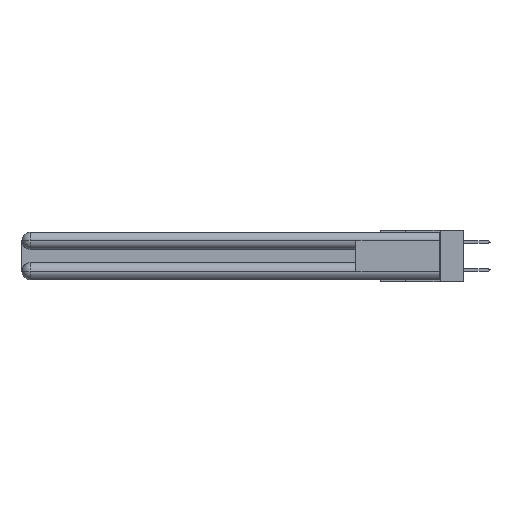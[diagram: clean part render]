
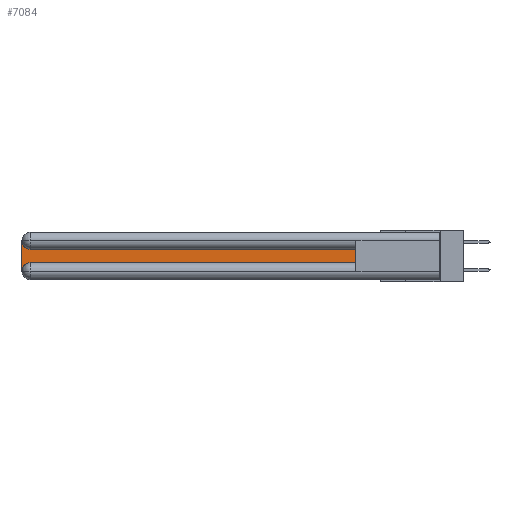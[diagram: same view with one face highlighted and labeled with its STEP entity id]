
A CAD part, left-side view. The second image highlights one B-rep face of the part: STEP entity #7084.
In plain terms, the highlighted planar face has unit normal (-1, 0, 0).
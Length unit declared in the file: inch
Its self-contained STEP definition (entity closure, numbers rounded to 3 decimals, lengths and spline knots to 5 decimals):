
#772 = ORIENTED_EDGE ( 'NONE', *, *, #11521, .T. ) ;
#3946 = VECTOR ( 'NONE', #28432, 39.37008 ) ;
#5142 = CIRCLE ( 'NONE', #7296, 0.06 ) ;
#6500 = DIRECTION ( 'NONE',  ( 0., 1., 0. ) ) ;
#7084 = ADVANCED_FACE ( 'NONE', ( #16347 ), #7309, .F. ) ;
#7296 = AXIS2_PLACEMENT_3D ( 'NONE', #9101, #19307, #32123 ) ;
#7309 = PLANE ( 'NONE',  #29893 ) ;
#7628 = EDGE_LOOP ( 'NONE', ( #17224, #16325, #29909, #25573, #772, #27453 ) ) ;
#9101 = CARTESIAN_POINT ( 'NONE',  ( 0.075, 2.94, -0.0625 ) ) ;
#9223 = EDGE_CURVE ( 'NONE', #13386, #19911, #5142, .T. ) ;
#9277 = EDGE_CURVE ( 'NONE', #19240, #13386, #19748, .T. ) ;
#9415 = EDGE_CURVE ( 'NONE', #11434, #25570, #26625, .T. ) ;
#9767 = CARTESIAN_POINT ( 'NONE',  ( 0.075, 0.6, -0.2175 ) ) ;
#10267 = VECTOR ( 'NONE', #27916, 39.37008 ) ;
#11434 = VERTEX_POINT ( 'NONE', #15117 ) ;
#11521 = EDGE_CURVE ( 'NONE', #25570, #14764, #17181, .T. ) ;
#11588 = EDGE_CURVE ( 'NONE', #19911, #11434, #22032, .T. ) ;
#12246 = DIRECTION ( 'NONE',  ( 0., 0., -1. ) ) ;
#12502 = CARTESIAN_POINT ( 'NONE',  ( 0.075, 3., -0.2175 ) ) ;
#12539 = DIRECTION ( 'NONE',  ( 0., 0., -1. ) ) ;
#13386 = VERTEX_POINT ( 'NONE', #27143 ) ;
#14418 = CARTESIAN_POINT ( 'NONE',  ( 0.075, 0.6, -0.1225 ) ) ;
#14764 = VERTEX_POINT ( 'NONE', #29469 ) ;
#15116 = DIRECTION ( 'NONE',  ( 0., 0., -1. ) ) ;
#15117 = CARTESIAN_POINT ( 'NONE',  ( 0.075, 3., -0.2775 ) ) ;
#16325 = ORIENTED_EDGE ( 'NONE', *, *, #9223, .T. ) ;
#16347 = FACE_OUTER_BOUND ( 'NONE', #7628, .T. ) ;
#17181 = LINE ( 'NONE', #9767, #10267 ) ;
#17224 = ORIENTED_EDGE ( 'NONE', *, *, #9277, .T. ) ;
#18053 = CARTESIAN_POINT ( 'NONE',  ( 0.075, 2.94, -0.2175 ) ) ;
#18393 = VECTOR ( 'NONE', #15116, 39.37008 ) ;
#19240 = VERTEX_POINT ( 'NONE', #21756 ) ;
#19307 = DIRECTION ( 'NONE',  ( 1., 0., 0. ) ) ;
#19748 = LINE ( 'NONE', #14418, #31117 ) ;
#19911 = VERTEX_POINT ( 'NONE', #25309 ) ;
#21756 = CARTESIAN_POINT ( 'NONE',  ( 0.075, 0.6, -0.1225 ) ) ;
#22032 = LINE ( 'NONE', #12502, #18393 ) ;
#23601 = AXIS2_PLACEMENT_3D ( 'NONE', #30072, #30182, #12246 ) ;
#23802 = EDGE_CURVE ( 'NONE', #14764, #19240, #33493, .T. ) ;
#25309 = CARTESIAN_POINT ( 'NONE',  ( 0.075, 3., -0.0625 ) ) ;
#25570 = VERTEX_POINT ( 'NONE', #18053 ) ;
#25573 = ORIENTED_EDGE ( 'NONE', *, *, #9415, .T. ) ;
#26625 = CIRCLE ( 'NONE', #23601, 0.06 ) ;
#27143 = CARTESIAN_POINT ( 'NONE',  ( 0.075, 2.94, -0.1225 ) ) ;
#27453 = ORIENTED_EDGE ( 'NONE', *, *, #23802, .T. ) ;
#27916 = DIRECTION ( 'NONE',  ( 0., -1., 0. ) ) ;
#28052 = DIRECTION ( 'NONE',  ( 1., 0., 0. ) ) ;
#28432 = DIRECTION ( 'NONE',  ( 0., 0., 1. ) ) ;
#29469 = CARTESIAN_POINT ( 'NONE',  ( 0.075, 0.6, -0.2175 ) ) ;
#29893 = AXIS2_PLACEMENT_3D ( 'NONE', #30916, #28052, #12539 ) ;
#29909 = ORIENTED_EDGE ( 'NONE', *, *, #11588, .T. ) ;
#30072 = CARTESIAN_POINT ( 'NONE',  ( 0.075, 2.94, -0.2775 ) ) ;
#30182 = DIRECTION ( 'NONE',  ( 1., 0., 0. ) ) ;
#30916 = CARTESIAN_POINT ( 'NONE',  ( 0.075, 3., -0.1225 ) ) ;
#30934 = CARTESIAN_POINT ( 'NONE',  ( 0.075, 0.6, -0.2175 ) ) ;
#31117 = VECTOR ( 'NONE', #6500, 39.37008 ) ;
#32123 = DIRECTION ( 'NONE',  ( 0., 0., -1. ) ) ;
#33493 = LINE ( 'NONE', #30934, #3946 ) ;
